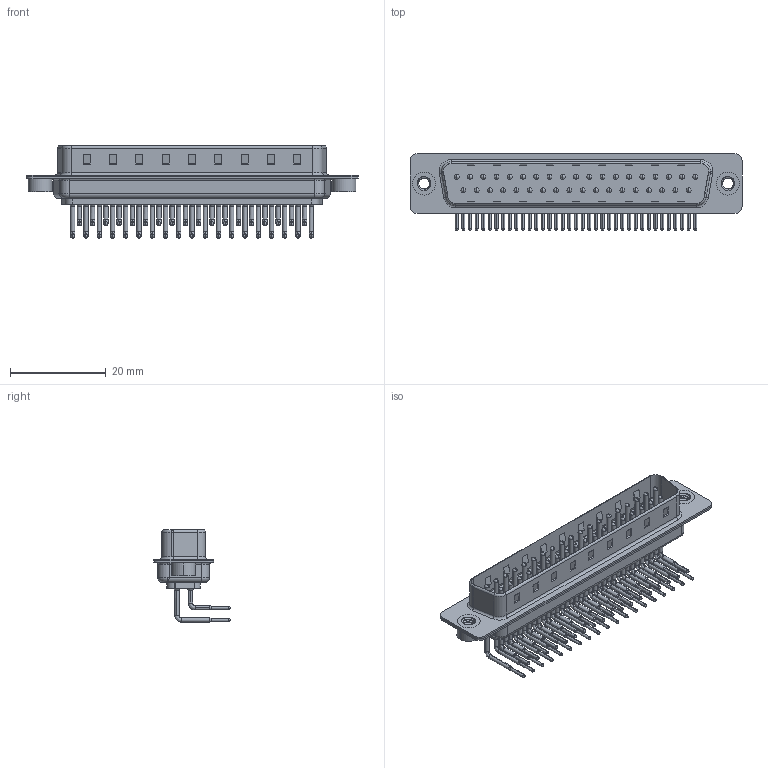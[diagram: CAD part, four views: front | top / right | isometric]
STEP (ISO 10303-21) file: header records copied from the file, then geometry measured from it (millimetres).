
FILE_DESCRIPTION (( 'STEP AP203' ), '1' );
FILE_NAME ('629-M37-340-LN2.STEP', '2018-09-25T22:15:41', ( '' ), ( '' ), 'SwSTEP 2.0', 'SolidWorks 2016', '' );
FILE_SCHEMA (( 'CONFIG_CONTROL_DESIGN' ));
Length unit declared in the file: millimetre
Products named in the file (7): 629M 4-40 Threaded Rivet; 629-M37-340-LN2; 629M Housing_37 Contacts; 629M Shell Front_37 Contacts; 629M Shell Rear_37 Contacts; 629M Contact Row 1; 629M Contact Row 2
Assembly tree (42 placements, depth 2):
  629-M37-340-LN2
    629M Housing_37 Contacts
    629M Shell Front_37 Contacts
    629M Shell Rear_37 Contacts
    629M Contact Row 1  x19
    629M Contact Row 2  x18
    629M 4-40 Threaded Rivet  x2
Bounding box: 69.4 x 16 x 19.29 mm (x, y, z)
Volume: 4051.2 mm3; surface area: 10619.7 mm2
Topology: 42 solids, 42 shells, 4482 faces, 12567 edges, 8180 vertices
Faces by surface type: plane 2571, cylinder 1473, bspline 228, cone 154, torus 56
Entity records: 30264 total; most frequent: CARTESIAN_POINT 6332, DIRECTION 4883, ORIENTED_EDGE 4442, EDGE_CURVE 2221, AXIS2_PLACEMENT_3D 1802, VERTEX_POINT 1441, VECTOR 1279, LINE 1279
